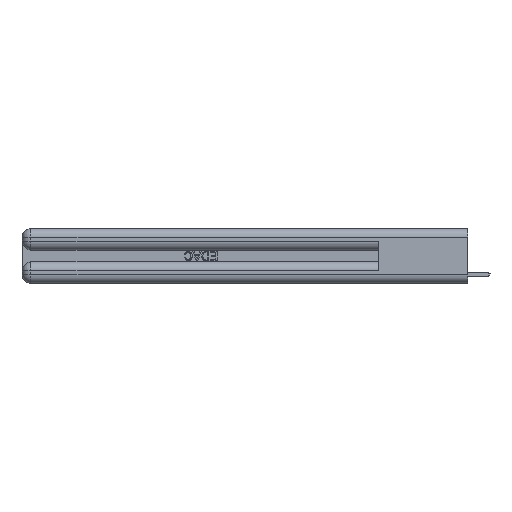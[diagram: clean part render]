
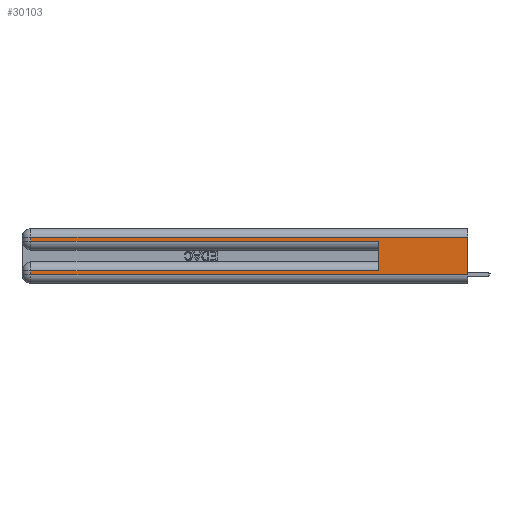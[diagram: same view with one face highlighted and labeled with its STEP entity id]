
A CAD part, left-side view. The second image highlights one B-rep face of the part: STEP entity #30103.
In plain terms, the highlighted planar face has unit normal (-1, 0, 0).
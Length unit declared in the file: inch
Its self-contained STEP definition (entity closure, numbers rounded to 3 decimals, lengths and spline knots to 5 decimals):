
#150 = LINE ( 'NONE', #5406, #16993 ) ;
#459 = EDGE_CURVE ( 'NONE', #26170, #32609, #26454, .T. ) ;
#491 = CARTESIAN_POINT ( 'NONE',  ( 0., 0., 0.37 ) ) ;
#1434 = ORIENTED_EDGE ( 'NONE', *, *, #459, .T. ) ;
#1553 = VERTEX_POINT ( 'NONE', #29352 ) ;
#1660 = VERTEX_POINT ( 'NONE', #12441 ) ;
#1966 = DIRECTION ( 'NONE',  ( 0., 0., -1. ) ) ;
#2070 = VECTOR ( 'NONE', #10919, 39.37008 ) ;
#2995 = CARTESIAN_POINT ( 'NONE',  ( 0., 0., 0.06 ) ) ;
#3099 = CARTESIAN_POINT ( 'NONE',  ( 0., 0., 0.06 ) ) ;
#3448 = DIRECTION ( 'NONE',  ( 0., -1., 0. ) ) ;
#3545 = DIRECTION ( 'NONE',  ( 0., 0., -1. ) ) ;
#3652 = VECTOR ( 'NONE', #12763, 39.37008 ) ;
#3702 = DIRECTION ( 'NONE',  ( 0., 0., -1. ) ) ;
#4181 = EDGE_LOOP ( 'NONE', ( #5507, #29370, #16241, #32262, #23219, #31108, #17292, #1434 ) ) ;
#4593 = CARTESIAN_POINT ( 'NONE',  ( 0., 2.94, 0.37 ) ) ;
#4833 = LINE ( 'NONE', #17964, #30453 ) ;
#5292 = EDGE_CURVE ( 'NONE', #27649, #7582, #19804, .T. ) ;
#5406 = CARTESIAN_POINT ( 'NONE',  ( 0., 0.6, 0.145 ) ) ;
#5507 = ORIENTED_EDGE ( 'NONE', *, *, #9455, .F. ) ;
#6191 = CARTESIAN_POINT ( 'NONE',  ( 0., 2.94, 0.31 ) ) ;
#6923 = LINE ( 'NONE', #24508, #32829 ) ;
#7391 = VERTEX_POINT ( 'NONE', #26899 ) ;
#7397 = DIRECTION ( 'NONE',  ( 1., 0., 0. ) ) ;
#7582 = VERTEX_POINT ( 'NONE', #28258 ) ;
#7802 = CARTESIAN_POINT ( 'NONE',  ( 0., 0.6, 0.085 ) ) ;
#8248 = EDGE_CURVE ( 'NONE', #7582, #26170, #6923, .T. ) ;
#9455 = EDGE_CURVE ( 'NONE', #7391, #32609, #16669, .T. ) ;
#9961 = FACE_OUTER_BOUND ( 'NONE', #4181, .T. ) ;
#10413 = CARTESIAN_POINT ( 'NONE',  ( 0., 2.94, 0.06 ) ) ;
#10919 = DIRECTION ( 'NONE',  ( 0., -1., 0. ) ) ;
#12441 = CARTESIAN_POINT ( 'NONE',  ( 0., 2.94, 0.285 ) ) ;
#12763 = DIRECTION ( 'NONE',  ( 0., 0., -1. ) ) ;
#15411 = VECTOR ( 'NONE', #3545, 39.37008 ) ;
#16241 = ORIENTED_EDGE ( 'NONE', *, *, #32007, .T. ) ;
#16460 = VECTOR ( 'NONE', #3448, 39.37008 ) ;
#16669 = LINE ( 'NONE', #491, #15411 ) ;
#16993 = VECTOR ( 'NONE', #23331, 39.37008 ) ;
#17085 = DIRECTION ( 'NONE',  ( 0., 1., 0. ) ) ;
#17292 = ORIENTED_EDGE ( 'NONE', *, *, #8248, .T. ) ;
#17903 = VERTEX_POINT ( 'NONE', #6191 ) ;
#17964 = CARTESIAN_POINT ( 'NONE',  ( 0., 0., 0.31 ) ) ;
#19804 = LINE ( 'NONE', #26804, #26195 ) ;
#20026 = PLANE ( 'NONE',  #30306 ) ;
#20778 = EDGE_CURVE ( 'NONE', #7391, #17903, #4833, .T. ) ;
#21723 = EDGE_CURVE ( 'NONE', #27649, #1553, #150, .T. ) ;
#22411 = CARTESIAN_POINT ( 'NONE',  ( 0., 0., 0.37 ) ) ;
#23219 = ORIENTED_EDGE ( 'NONE', *, *, #21723, .F. ) ;
#23331 = DIRECTION ( 'NONE',  ( 0., 0., 1. ) ) ;
#24508 = CARTESIAN_POINT ( 'NONE',  ( 0., 2.94, 0.37 ) ) ;
#24626 = EDGE_CURVE ( 'NONE', #1660, #1553, #32079, .T. ) ;
#26170 = VERTEX_POINT ( 'NONE', #10413 ) ;
#26195 = VECTOR ( 'NONE', #17085, 39.37008 ) ;
#26454 = LINE ( 'NONE', #3099, #2070 ) ;
#26804 = CARTESIAN_POINT ( 'NONE',  ( 0., 0., 0.085 ) ) ;
#26899 = CARTESIAN_POINT ( 'NONE',  ( 0., 0., 0.31 ) ) ;
#27144 = CARTESIAN_POINT ( 'NONE',  ( 0., 0., 0.285 ) ) ;
#27649 = VERTEX_POINT ( 'NONE', #7802 ) ;
#28258 = CARTESIAN_POINT ( 'NONE',  ( 0., 2.94, 0.085 ) ) ;
#28370 = DIRECTION ( 'NONE',  ( 0., 1., 0. ) ) ;
#29352 = CARTESIAN_POINT ( 'NONE',  ( 0., 0.6, 0.285 ) ) ;
#29370 = ORIENTED_EDGE ( 'NONE', *, *, #20778, .T. ) ;
#30103 = ADVANCED_FACE ( 'NONE', ( #9961 ), #20026, .F. ) ;
#30306 = AXIS2_PLACEMENT_3D ( 'NONE', #22411, #7397, #1966 ) ;
#30453 = VECTOR ( 'NONE', #28370, 39.37008 ) ;
#30844 = LINE ( 'NONE', #4593, #3652 ) ;
#31108 = ORIENTED_EDGE ( 'NONE', *, *, #5292, .T. ) ;
#32007 = EDGE_CURVE ( 'NONE', #17903, #1660, #30844, .T. ) ;
#32079 = LINE ( 'NONE', #27144, #16460 ) ;
#32262 = ORIENTED_EDGE ( 'NONE', *, *, #24626, .T. ) ;
#32609 = VERTEX_POINT ( 'NONE', #2995 ) ;
#32829 = VECTOR ( 'NONE', #3702, 39.37008 ) ;
